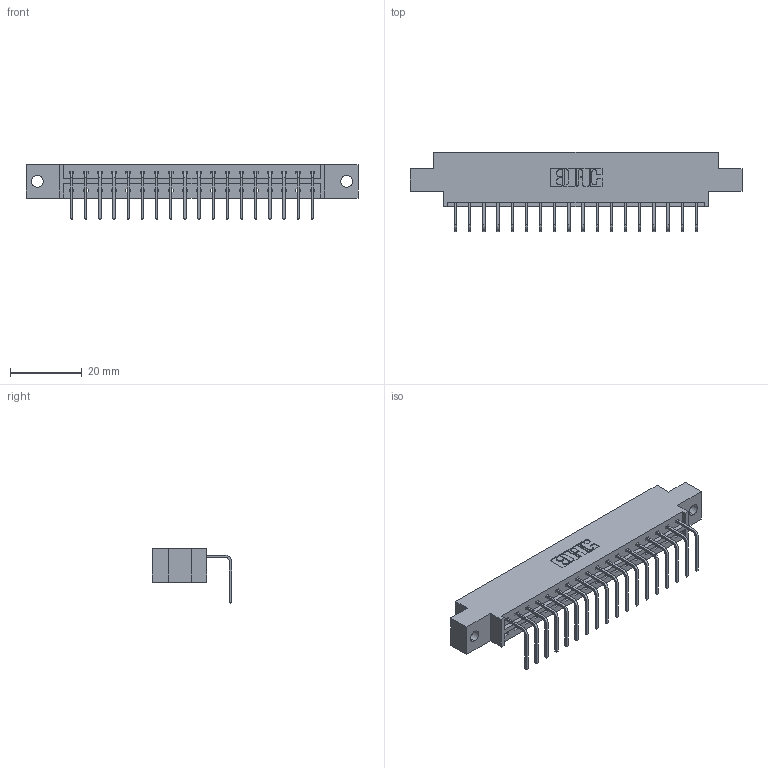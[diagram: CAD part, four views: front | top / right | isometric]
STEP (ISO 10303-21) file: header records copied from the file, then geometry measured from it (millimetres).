
FILE_DESCRIPTION (( 'STEP AP203' ), '1' );
FILE_NAME ('333-018-558-602.STEP', '2019-08-09T14:12:27', ( '' ), ( '' ), 'SwSTEP 2.0', 'SolidWorks 2016', '' );
FILE_SCHEMA (( 'CONFIG_CONTROL_DESIGN' ));
Length unit declared in the file: inch
Products named in the file (3): 333-018-558-602; 345-292-001_558 Tail - 2; 333 Part_Offset - .128 Dia
Assembly tree (19 placements, depth 2):
  333-018-558-602
    333 Part_Offset - .128 Dia
    345-292-001_558 Tail - 2  x18
Bounding box: 92.86 x 22.17 x 15.37 mm (x, y, z)
Volume: 8933.7 mm3; surface area: 9802.5 mm2
Topology: 19 solids, 19 shells, 1198 faces, 3599 edges, 2374 vertices
Faces by surface type: plane 866, cylinder 332
Entity records: 14327 total; most frequent: CARTESIAN_POINT 2484, ORIENTED_EDGE 2438, DIRECTION 2143, EDGE_CURVE 1219, LINE 1091, VECTOR 1091, VERTEX_POINT 810, AXIS2_PLACEMENT_3D 526
